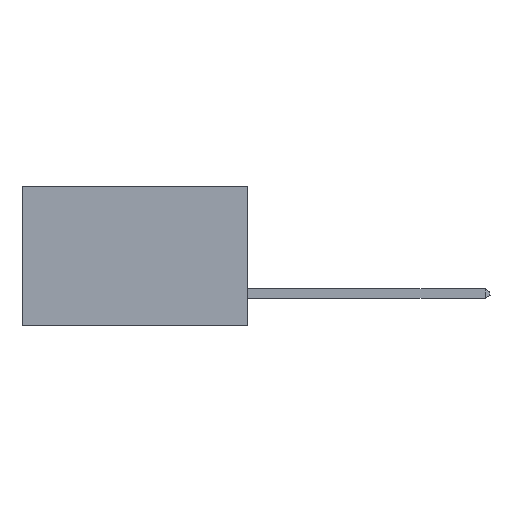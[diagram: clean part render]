
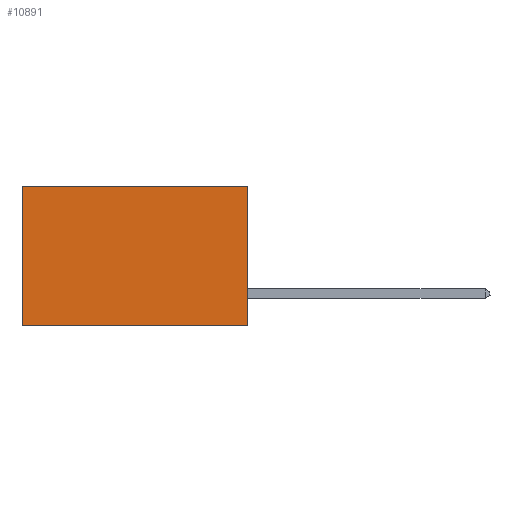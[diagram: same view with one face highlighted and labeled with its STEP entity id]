
A CAD part, left-side view. The second image highlights one B-rep face of the part: STEP entity #10891.
In plain terms, the highlighted planar face has unit normal (-1, 0, 0).
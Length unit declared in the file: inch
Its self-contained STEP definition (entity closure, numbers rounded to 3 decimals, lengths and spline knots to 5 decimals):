
#131 = VERTEX_POINT ( 'NONE', #7456 ) ;
#1078 = CARTESIAN_POINT ( 'NONE',  ( 0.298, 0.6, 0. ) ) ;
#1351 = LINE ( 'NONE', #10746, #4366 ) ;
#1448 = VERTEX_POINT ( 'NONE', #9149 ) ;
#1881 = VERTEX_POINT ( 'NONE', #10619 ) ;
#2130 = DIRECTION ( 'NONE',  ( 1., 0., 0. ) ) ;
#2267 = EDGE_CURVE ( 'NONE', #1881, #131, #1351, .T. ) ;
#2780 = ORIENTED_EDGE ( 'NONE', *, *, #7372, .F. ) ;
#3098 = DIRECTION ( 'NONE',  ( 0., 0., -1. ) ) ;
#3399 = ORIENTED_EDGE ( 'NONE', *, *, #2267, .F. ) ;
#3546 = EDGE_CURVE ( 'NONE', #8415, #1448, #7107, .T. ) ;
#3757 = DIRECTION ( 'NONE',  ( 0., 1., 0. ) ) ;
#3879 = AXIS2_PLACEMENT_3D ( 'NONE', #7900, #2130, #3098 ) ;
#4014 = PLANE ( 'NONE',  #3879 ) ;
#4366 = VECTOR ( 'NONE', #11714, 39.37008 ) ;
#4587 = LINE ( 'NONE', #4688, #7303 ) ;
#4688 = CARTESIAN_POINT ( 'NONE',  ( 0.298, 0., 0. ) ) ;
#4852 = VECTOR ( 'NONE', #8177, 39.37008 ) ;
#4895 = LINE ( 'NONE', #6881, #9860 ) ;
#6393 = EDGE_LOOP ( 'NONE', ( #7572, #2780, #3399, #12000 ) ) ;
#6790 = EDGE_CURVE ( 'NONE', #1881, #8415, #4587, .T. ) ;
#6881 = CARTESIAN_POINT ( 'NONE',  ( 0.298, 0., -0.37 ) ) ;
#7107 = LINE ( 'NONE', #8257, #4852 ) ;
#7303 = VECTOR ( 'NONE', #3757, 39.37008 ) ;
#7372 = EDGE_CURVE ( 'NONE', #131, #1448, #4895, .T. ) ;
#7456 = CARTESIAN_POINT ( 'NONE',  ( 0.298, 0., -0.37 ) ) ;
#7572 = ORIENTED_EDGE ( 'NONE', *, *, #3546, .T. ) ;
#7837 = DIRECTION ( 'NONE',  ( 0., 1., 0. ) ) ;
#7900 = CARTESIAN_POINT ( 'NONE',  ( 0.298, 0., 0. ) ) ;
#8177 = DIRECTION ( 'NONE',  ( 0., 0., -1. ) ) ;
#8257 = CARTESIAN_POINT ( 'NONE',  ( 0.298, 0.6, 0. ) ) ;
#8415 = VERTEX_POINT ( 'NONE', #1078 ) ;
#9149 = CARTESIAN_POINT ( 'NONE',  ( 0.298, 0.6, -0.37 ) ) ;
#9860 = VECTOR ( 'NONE', #7837, 39.37008 ) ;
#10619 = CARTESIAN_POINT ( 'NONE',  ( 0.298, 0., 0. ) ) ;
#10746 = CARTESIAN_POINT ( 'NONE',  ( 0.298, 0., 0. ) ) ;
#10891 = ADVANCED_FACE ( 'NONE', ( #12413 ), #4014, .F. ) ;
#11714 = DIRECTION ( 'NONE',  ( 0., 0., -1. ) ) ;
#12000 = ORIENTED_EDGE ( 'NONE', *, *, #6790, .T. ) ;
#12413 = FACE_OUTER_BOUND ( 'NONE', #6393, .T. ) ;
